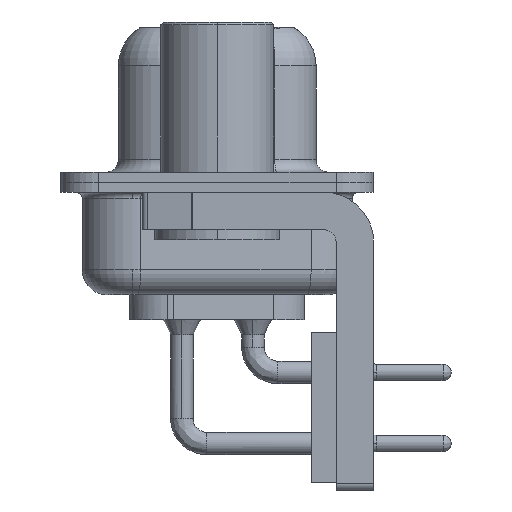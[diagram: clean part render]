
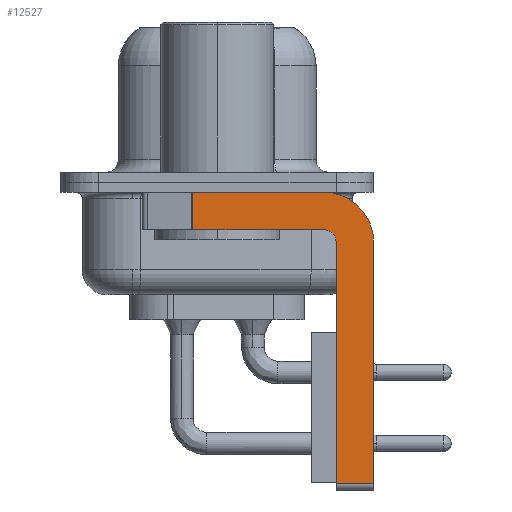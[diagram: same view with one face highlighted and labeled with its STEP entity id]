
A CAD part, left-side view. The second image highlights one B-rep face of the part: STEP entity #12527.
In plain terms, the highlighted planar face has unit normal (-1, 0, 0).
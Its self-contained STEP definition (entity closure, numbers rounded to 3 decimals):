
#473 = VERTEX_POINT ( 'NONE', #5618 ) ;
#1001 = DIRECTION ( 'NONE',  ( 0., 0., 1. ) ) ;
#1415 = VERTEX_POINT ( 'NONE', #15797 ) ;
#2776 = ORIENTED_EDGE ( 'NONE', *, *, #15967, .F. ) ;
#3546 = ORIENTED_EDGE ( 'NONE', *, *, #24474, .F. ) ;
#3594 = EDGE_LOOP ( 'NONE', ( #2776, #28466, #17228, #18706, #20974, #26995, #3546, #8514 ) ) ;
#3869 = AXIS2_PLACEMENT_3D ( 'NONE', #30449, #15674, #1001 ) ;
#3931 = VERTEX_POINT ( 'NONE', #25284 ) ;
#4327 = CARTESIAN_POINT ( 'NONE',  ( -2.9, -4.25, -2.4 ) ) ;
#4421 = DIRECTION ( 'NONE',  ( 1., 0., 0. ) ) ;
#4431 = PLANE ( 'NONE',  #27218 ) ;
#5292 = CIRCLE ( 'NONE', #8569, 2. ) ;
#5477 = VECTOR ( 'NONE', #11831, 1000. ) ;
#5554 = CARTESIAN_POINT ( 'NONE',  ( -2.9, -4.75, -2.4 ) ) ;
#5618 = CARTESIAN_POINT ( 'NONE',  ( -2.9, -4.25, -0.4 ) ) ;
#5901 = DIRECTION ( 'NONE',  ( 0., 0., -1. ) ) ;
#6318 = EDGE_CURVE ( 'NONE', #27243, #1415, #13292, .T. ) ;
#7741 = EDGE_CURVE ( 'NONE', #23924, #26361, #17098, .T. ) ;
#8430 = VERTEX_POINT ( 'NONE', #20590 ) ;
#8514 = ORIENTED_EDGE ( 'NONE', *, *, #16514, .F. ) ;
#8569 = AXIS2_PLACEMENT_3D ( 'NONE', #19140, #4421, #21629 ) ;
#9319 = DIRECTION ( 'NONE',  ( 0., 0., -1. ) ) ;
#9352 = DIRECTION ( 'NONE',  ( 0., -1., 0. ) ) ;
#10165 = VECTOR ( 'NONE', #5901, 1000. ) ;
#10530 = EDGE_CURVE ( 'NONE', #8430, #3931, #29879, .T. ) ;
#11403 = CARTESIAN_POINT ( 'NONE',  ( -2.9, -4.75, -12.3 ) ) ;
#11831 = DIRECTION ( 'NONE',  ( 0., 1., 0. ) ) ;
#12221 = CARTESIAN_POINT ( 'NONE',  ( -2.9, -6.25, -2.4 ) ) ;
#12527 = ADVANCED_FACE ( 'NONE', ( #22451 ), #4431, .F. ) ;
#13099 = EDGE_CURVE ( 'NONE', #27243, #23924, #17390, .T. ) ;
#13292 = LINE ( 'NONE', #17172, #25617 ) ;
#13858 = CARTESIAN_POINT ( 'NONE',  ( -2.9, 3., -0.4 ) ) ;
#15674 = DIRECTION ( 'NONE',  ( -1., 0., 0. ) ) ;
#15797 = CARTESIAN_POINT ( 'NONE',  ( -2.9, -6.25, -12.05 ) ) ;
#15967 = EDGE_CURVE ( 'NONE', #8430, #473, #30750, .T. ) ;
#16392 = DIRECTION ( 'NONE',  ( 0., 0., 1. ) ) ;
#16514 = EDGE_CURVE ( 'NONE', #473, #30857, #5292, .T. ) ;
#17079 = DIRECTION ( 'NONE',  ( 0., -1., 0. ) ) ;
#17098 = CIRCLE ( 'NONE', #3869, 0.5 ) ;
#17172 = CARTESIAN_POINT ( 'NONE',  ( -2.9, -4.25, -12.05 ) ) ;
#17228 = ORIENTED_EDGE ( 'NONE', *, *, #29997, .F. ) ;
#17390 = LINE ( 'NONE', #11403, #23175 ) ;
#18706 = ORIENTED_EDGE ( 'NONE', *, *, #7741, .F. ) ;
#19140 = CARTESIAN_POINT ( 'NONE',  ( -2.9, -4.25, -2.4 ) ) ;
#20590 = CARTESIAN_POINT ( 'NONE',  ( -2.9, 0.978, -0.4 ) ) ;
#20974 = ORIENTED_EDGE ( 'NONE', *, *, #13099, .F. ) ;
#21629 = DIRECTION ( 'NONE',  ( 0., 0., -1. ) ) ;
#22336 = VECTOR ( 'NONE', #30922, 1000. ) ;
#22451 = FACE_OUTER_BOUND ( 'NONE', #3594, .T. ) ;
#23115 = CARTESIAN_POINT ( 'NONE',  ( -2.9, 0.978, -1.9 ) ) ;
#23175 = VECTOR ( 'NONE', #16392, 1000. ) ;
#23441 = CARTESIAN_POINT ( 'NONE',  ( -2.9, -6.25, -2.4 ) ) ;
#23924 = VERTEX_POINT ( 'NONE', #5554 ) ;
#23971 = CARTESIAN_POINT ( 'NONE',  ( -2.9, -4.25, -1.9 ) ) ;
#24063 = DIRECTION ( 'NONE',  ( 1., 0., 0. ) ) ;
#24474 = EDGE_CURVE ( 'NONE', #30857, #1415, #28861, .T. ) ;
#25284 = CARTESIAN_POINT ( 'NONE',  ( -2.9, 0.978, -1.9 ) ) ;
#25617 = VECTOR ( 'NONE', #17079, 1000. ) ;
#26361 = VERTEX_POINT ( 'NONE', #23971 ) ;
#26600 = CARTESIAN_POINT ( 'NONE',  ( -2.9, -4.25, -1.9 ) ) ;
#26995 = ORIENTED_EDGE ( 'NONE', *, *, #6318, .T. ) ;
#27218 = AXIS2_PLACEMENT_3D ( 'NONE', #4327, #24063, #9319 ) ;
#27243 = VERTEX_POINT ( 'NONE', #30216 ) ;
#28466 = ORIENTED_EDGE ( 'NONE', *, *, #10530, .T. ) ;
#28861 = LINE ( 'NONE', #23441, #22336 ) ;
#29879 = LINE ( 'NONE', #23115, #10165 ) ;
#29960 = VECTOR ( 'NONE', #9352, 1000. ) ;
#29997 = EDGE_CURVE ( 'NONE', #26361, #3931, #31702, .T. ) ;
#30216 = CARTESIAN_POINT ( 'NONE',  ( -2.9, -4.75, -12.05 ) ) ;
#30449 = CARTESIAN_POINT ( 'NONE',  ( -2.9, -4.25, -2.4 ) ) ;
#30750 = LINE ( 'NONE', #13858, #29960 ) ;
#30857 = VERTEX_POINT ( 'NONE', #12221 ) ;
#30922 = DIRECTION ( 'NONE',  ( 0., 0., -1. ) ) ;
#31702 = LINE ( 'NONE', #26600, #5477 ) ;
